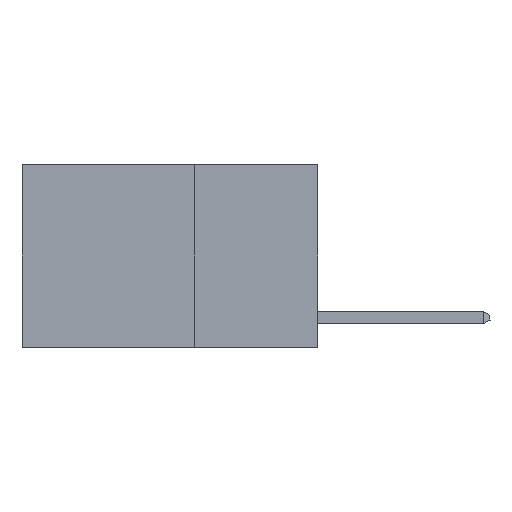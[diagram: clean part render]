
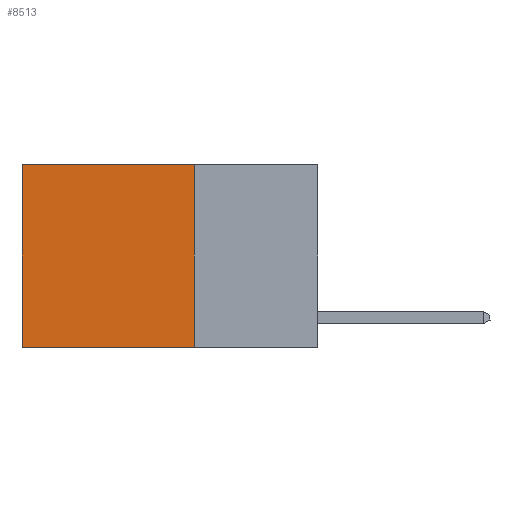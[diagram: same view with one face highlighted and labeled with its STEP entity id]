
A CAD part, left-side view. The second image highlights one B-rep face of the part: STEP entity #8513.
In plain terms, the highlighted planar face has unit normal (-1, 0, 0).
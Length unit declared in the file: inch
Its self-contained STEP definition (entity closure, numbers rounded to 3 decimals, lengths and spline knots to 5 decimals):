
#278 = ORIENTED_EDGE ( 'NONE', *, *, #21043, .T. ) ;
#283 = CARTESIAN_POINT ( 'NONE',  ( 0.2625, 0.25, 0. ) ) ;
#1429 = CARTESIAN_POINT ( 'NONE',  ( 0.2625, 0.25, -0.37 ) ) ;
#1627 = FACE_OUTER_BOUND ( 'NONE', #15984, .T. ) ;
#2768 = VERTEX_POINT ( 'NONE', #7666 ) ;
#3868 = EDGE_CURVE ( 'NONE', #7400, #16190, #14766, .T. ) ;
#4613 = VECTOR ( 'NONE', #12741, 39.37008 ) ;
#4852 = AXIS2_PLACEMENT_3D ( 'NONE', #5108, #17123, #6849 ) ;
#5108 = CARTESIAN_POINT ( 'NONE',  ( 0.2625, 0.25, 0. ) ) ;
#5247 = CARTESIAN_POINT ( 'NONE',  ( 0.2625, 0.6, -0.37 ) ) ;
#6282 = CARTESIAN_POINT ( 'NONE',  ( 0.2625, 0.6, 0. ) ) ;
#6657 = VERTEX_POINT ( 'NONE', #283 ) ;
#6849 = DIRECTION ( 'NONE',  ( 0., 0., -1. ) ) ;
#7400 = VERTEX_POINT ( 'NONE', #9082 ) ;
#7666 = CARTESIAN_POINT ( 'NONE',  ( 0.2625, 0.6, 0. ) ) ;
#8152 = EDGE_CURVE ( 'NONE', #6657, #7400, #9191, .T. ) ;
#8513 = ADVANCED_FACE ( 'NONE', ( #1627 ), #15405, .F. ) ;
#8589 = VECTOR ( 'NONE', #19998, 39.37008 ) ;
#9082 = CARTESIAN_POINT ( 'NONE',  ( 0.2625, 0.25, -0.37 ) ) ;
#9134 = LINE ( 'NONE', #14833, #8589 ) ;
#9191 = LINE ( 'NONE', #21242, #4613 ) ;
#9443 = EDGE_CURVE ( 'NONE', #6657, #2768, #9134, .T. ) ;
#9504 = ORIENTED_EDGE ( 'NONE', *, *, #3868, .F. ) ;
#10191 = VECTOR ( 'NONE', #15185, 39.37008 ) ;
#11672 = VECTOR ( 'NONE', #13202, 39.37008 ) ;
#11719 = ORIENTED_EDGE ( 'NONE', *, *, #8152, .F. ) ;
#12741 = DIRECTION ( 'NONE',  ( 0., 0., -1. ) ) ;
#13202 = DIRECTION ( 'NONE',  ( 0., 0., -1. ) ) ;
#14766 = LINE ( 'NONE', #1429, #10191 ) ;
#14833 = CARTESIAN_POINT ( 'NONE',  ( 0.2625, 0.25, 0. ) ) ;
#15185 = DIRECTION ( 'NONE',  ( 0., 1., 0. ) ) ;
#15405 = PLANE ( 'NONE',  #4852 ) ;
#15984 = EDGE_LOOP ( 'NONE', ( #278, #9504, #11719, #18656 ) ) ;
#16190 = VERTEX_POINT ( 'NONE', #5247 ) ;
#16214 = LINE ( 'NONE', #6282, #11672 ) ;
#17123 = DIRECTION ( 'NONE',  ( 1., 0., 0. ) ) ;
#18656 = ORIENTED_EDGE ( 'NONE', *, *, #9443, .T. ) ;
#19998 = DIRECTION ( 'NONE',  ( 0., 1., 0. ) ) ;
#21043 = EDGE_CURVE ( 'NONE', #2768, #16190, #16214, .T. ) ;
#21242 = CARTESIAN_POINT ( 'NONE',  ( 0.2625, 0.25, 0. ) ) ;
